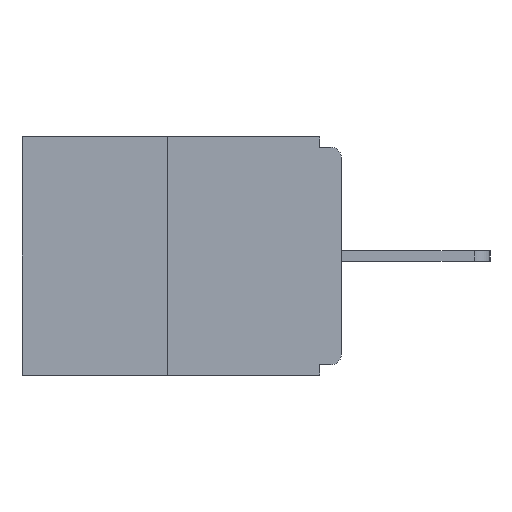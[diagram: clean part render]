
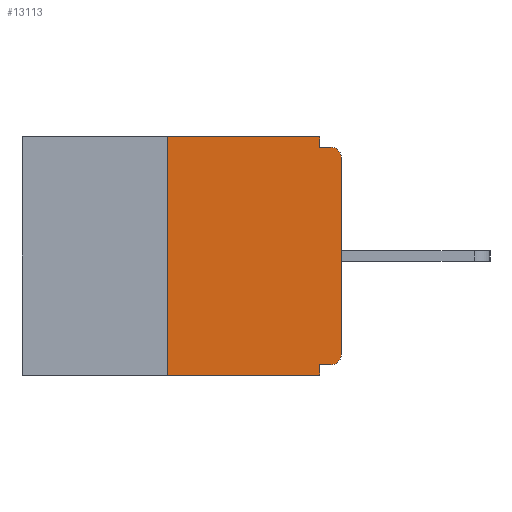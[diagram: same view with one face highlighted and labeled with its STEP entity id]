
A CAD part, left-side view. The second image highlights one B-rep face of the part: STEP entity #13113.
In plain terms, the highlighted planar face has unit normal (-1, 0, 0).
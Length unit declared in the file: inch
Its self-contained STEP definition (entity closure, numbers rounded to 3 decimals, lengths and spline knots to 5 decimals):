
#1141 = LINE ( 'NONE', #9400, #12062 ) ;
#1483 = VERTEX_POINT ( 'NONE', #6125 ) ;
#1780 = CARTESIAN_POINT ( 'NONE',  ( 0., 0.015, -0.328 ) ) ;
#1834 = CARTESIAN_POINT ( 'NONE',  ( 0., 0.031, -0.343 ) ) ;
#2245 = EDGE_CURVE ( 'NONE', #2971, #23837, #14598, .T. ) ;
#2971 = VERTEX_POINT ( 'NONE', #1780 ) ;
#3188 = DIRECTION ( 'NONE',  ( 0., -1., 0. ) ) ;
#3436 = DIRECTION ( 'NONE',  ( 0., 1., 0. ) ) ;
#4528 = ORIENTED_EDGE ( 'NONE', *, *, #21756, .T. ) ;
#5556 = ORIENTED_EDGE ( 'NONE', *, *, #12427, .T. ) ;
#5762 = CARTESIAN_POINT ( 'NONE',  ( 0., 0.031, -0.343 ) ) ;
#5915 = ORIENTED_EDGE ( 'NONE', *, *, #24425, .T. ) ;
#6125 = CARTESIAN_POINT ( 'NONE',  ( 0., 0., -0.03 ) ) ;
#6600 = ORIENTED_EDGE ( 'NONE', *, *, #10854, .F. ) ;
#7647 = ORIENTED_EDGE ( 'NONE', *, *, #2245, .F. ) ;
#7946 = EDGE_CURVE ( 'NONE', #25346, #23904, #27293, .T. ) ;
#8330 = EDGE_CURVE ( 'NONE', #23904, #18142, #1141, .T. ) ;
#8343 = LINE ( 'NONE', #20286, #19517 ) ;
#8965 = ORIENTED_EDGE ( 'NONE', *, *, #8330, .F. ) ;
#8995 = ORIENTED_EDGE ( 'NONE', *, *, #18090, .T. ) ;
#9400 = CARTESIAN_POINT ( 'NONE',  ( 0., 0.46, 0. ) ) ;
#9655 = CARTESIAN_POINT ( 'NONE',  ( 0., 0.46, 0. ) ) ;
#9915 = DIRECTION ( 'NONE',  ( 0., -1., 0. ) ) ;
#10491 = AXIS2_PLACEMENT_3D ( 'NONE', #11699, #26223, #13778 ) ;
#10508 = CARTESIAN_POINT ( 'NONE',  ( 0., 0.25, 0. ) ) ;
#10756 = DIRECTION ( 'NONE',  ( -1., 0., 0. ) ) ;
#10853 = CARTESIAN_POINT ( 'NONE',  ( 0., 0.015, -0.015 ) ) ;
#10854 = EDGE_CURVE ( 'NONE', #24739, #24457, #27445, .T. ) ;
#10869 = LINE ( 'NONE', #19940, #21319 ) ;
#11542 = VERTEX_POINT ( 'NONE', #1834 ) ;
#11699 = CARTESIAN_POINT ( 'NONE',  ( 0., 0.015, -0.313 ) ) ;
#11777 = DIRECTION ( 'NONE',  ( 0., 0., -1. ) ) ;
#12062 = VECTOR ( 'NONE', #9915, 39.37008 ) ;
#12236 = VECTOR ( 'NONE', #3188, 39.37008 ) ;
#12285 = VECTOR ( 'NONE', #20592, 39.37008 ) ;
#12427 = EDGE_CURVE ( 'NONE', #25346, #11542, #10869, .T. ) ;
#13014 = CARTESIAN_POINT ( 'NONE',  ( 0., 0., 0. ) ) ;
#13113 = ADVANCED_FACE ( 'NONE', ( #15580 ), #13764, .F. ) ;
#13584 = ORIENTED_EDGE ( 'NONE', *, *, #7946, .F. ) ;
#13764 = PLANE ( 'NONE',  #15660 ) ;
#13778 = DIRECTION ( 'NONE',  ( 0., 0., -1. ) ) ;
#14598 = LINE ( 'NONE', #16817, #19496 ) ;
#14617 = CARTESIAN_POINT ( 'NONE',  ( 0., 0., -0.313 ) ) ;
#15137 = DIRECTION ( 'NONE',  ( 0., 0., 1. ) ) ;
#15580 = FACE_OUTER_BOUND ( 'NONE', #25794, .T. ) ;
#15660 = AXIS2_PLACEMENT_3D ( 'NONE', #9655, #24250, #11777 ) ;
#16053 = CARTESIAN_POINT ( 'NONE',  ( 0., 0., -0.015 ) ) ;
#16817 = CARTESIAN_POINT ( 'NONE',  ( 0., 0., -0.328 ) ) ;
#17870 = ORIENTED_EDGE ( 'NONE', *, *, #26727, .F. ) ;
#18024 = CARTESIAN_POINT ( 'NONE',  ( 0., 0.25, -0.343 ) ) ;
#18090 = EDGE_CURVE ( 'NONE', #2971, #23871, #26639, .T. ) ;
#18142 = VERTEX_POINT ( 'NONE', #22289 ) ;
#18254 = DIRECTION ( 'NONE',  ( 0., 0., -1. ) ) ;
#19496 = VECTOR ( 'NONE', #3436, 39.37008 ) ;
#19517 = VECTOR ( 'NONE', #18254, 39.37008 ) ;
#19940 = CARTESIAN_POINT ( 'NONE',  ( 0., 0.46, -0.343 ) ) ;
#20286 = CARTESIAN_POINT ( 'NONE',  ( 0., 0.031, 0. ) ) ;
#20592 = DIRECTION ( 'NONE',  ( 0., 0., -1. ) ) ;
#20760 = CARTESIAN_POINT ( 'NONE',  ( 0., 0.031, -0.328 ) ) ;
#21200 = VECTOR ( 'NONE', #26503, 39.37008 ) ;
#21213 = AXIS2_PLACEMENT_3D ( 'NONE', #23257, #10756, #25316 ) ;
#21319 = VECTOR ( 'NONE', #22031, 39.37008 ) ;
#21756 = EDGE_CURVE ( 'NONE', #23871, #1483, #21840, .T. ) ;
#21840 = LINE ( 'NONE', #13014, #26650 ) ;
#22031 = DIRECTION ( 'NONE',  ( 0., -1., 0. ) ) ;
#22289 = CARTESIAN_POINT ( 'NONE',  ( 0., 0.031, 0. ) ) ;
#23257 = CARTESIAN_POINT ( 'NONE',  ( 0., 0.015, -0.03 ) ) ;
#23363 = LINE ( 'NONE', #5762, #12285 ) ;
#23658 = CIRCLE ( 'NONE', #21213, 0.015 ) ;
#23722 = ORIENTED_EDGE ( 'NONE', *, *, #23800, .F. ) ;
#23800 = EDGE_CURVE ( 'NONE', #23837, #11542, #23363, .T. ) ;
#23837 = VERTEX_POINT ( 'NONE', #20760 ) ;
#23871 = VERTEX_POINT ( 'NONE', #14617 ) ;
#23904 = VERTEX_POINT ( 'NONE', #10508 ) ;
#24250 = DIRECTION ( 'NONE',  ( 1., 0., 0. ) ) ;
#24419 = CARTESIAN_POINT ( 'NONE',  ( 0., 0.031, -0.015 ) ) ;
#24425 = EDGE_CURVE ( 'NONE', #1483, #24457, #23658, .T. ) ;
#24457 = VERTEX_POINT ( 'NONE', #10853 ) ;
#24739 = VERTEX_POINT ( 'NONE', #24419 ) ;
#25316 = DIRECTION ( 'NONE',  ( 0., 0., -1. ) ) ;
#25346 = VERTEX_POINT ( 'NONE', #18024 ) ;
#25794 = EDGE_LOOP ( 'NONE', ( #8965, #13584, #5556, #23722, #7647, #8995, #4528, #5915, #6600, #17870 ) ) ;
#26223 = DIRECTION ( 'NONE',  ( -1., 0., 0. ) ) ;
#26503 = DIRECTION ( 'NONE',  ( 0., 0., 1. ) ) ;
#26639 = CIRCLE ( 'NONE', #10491, 0.015 ) ;
#26650 = VECTOR ( 'NONE', #15137, 39.37008 ) ;
#26727 = EDGE_CURVE ( 'NONE', #18142, #24739, #8343, .T. ) ;
#26762 = CARTESIAN_POINT ( 'NONE',  ( 0., 0.25, 0. ) ) ;
#27293 = LINE ( 'NONE', #26762, #21200 ) ;
#27445 = LINE ( 'NONE', #16053, #12236 ) ;
